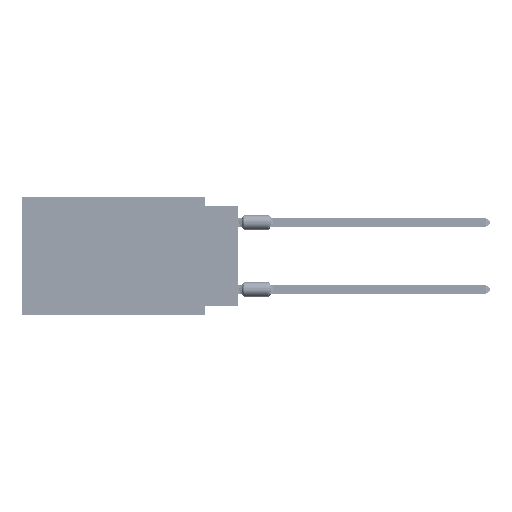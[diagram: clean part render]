
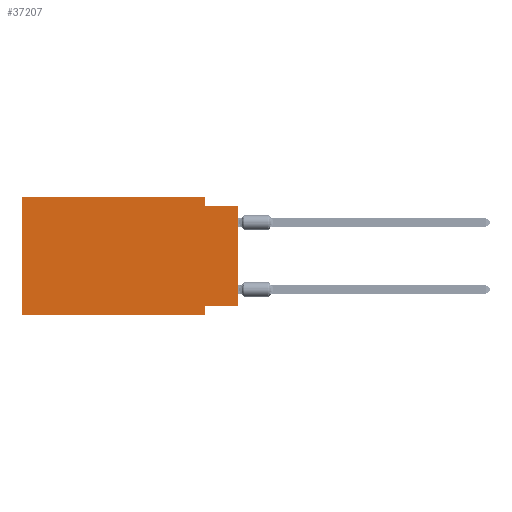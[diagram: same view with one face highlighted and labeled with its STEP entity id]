
A CAD part, left-side view. The second image highlights one B-rep face of the part: STEP entity #37207.
In plain terms, the highlighted planar face has unit normal (-1, 0, 0).
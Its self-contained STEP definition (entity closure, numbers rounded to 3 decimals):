
#640 = CARTESIAN_POINT ( 'NONE',  ( 0., 16.383, -8.89 ) ) ;
#1856 = VECTOR ( 'NONE', #93456, 1000. ) ;
#2628 = EDGE_CURVE ( 'NONE', #39612, #108847, #84671, .T. ) ;
#5478 = EDGE_CURVE ( 'NONE', #14094, #18456, #57519, .T. ) ;
#6122 = ORIENTED_EDGE ( 'NONE', *, *, #53269, .F. ) ;
#11257 = VERTEX_POINT ( 'NONE', #21645 ) ;
#11419 = CARTESIAN_POINT ( 'NONE',  ( 0., 16.383, 0. ) ) ;
#11695 = DIRECTION ( 'NONE',  ( 0., -1., 0. ) ) ;
#11996 = CARTESIAN_POINT ( 'NONE',  ( 0., 0., -8.255 ) ) ;
#14094 = VERTEX_POINT ( 'NONE', #640 ) ;
#14191 = VERTEX_POINT ( 'NONE', #103456 ) ;
#14547 = VECTOR ( 'NONE', #74507, 1000. ) ;
#17309 = VECTOR ( 'NONE', #94167, 1000. ) ;
#17633 = ORIENTED_EDGE ( 'NONE', *, *, #5478, .F. ) ;
#18456 = VERTEX_POINT ( 'NONE', #22431 ) ;
#19859 = CARTESIAN_POINT ( 'NONE',  ( 0., 16.383, 0. ) ) ;
#20325 = CARTESIAN_POINT ( 'NONE',  ( 0., 0., -0.635 ) ) ;
#20361 = CARTESIAN_POINT ( 'NONE',  ( 0., 0., -0.635 ) ) ;
#21645 = CARTESIAN_POINT ( 'NONE',  ( 0., 2.54, -8.89 ) ) ;
#22431 = CARTESIAN_POINT ( 'NONE',  ( 0., 16.383, 0. ) ) ;
#22819 = LINE ( 'NONE', #58480, #17309 ) ;
#27269 = ORIENTED_EDGE ( 'NONE', *, *, #110297, .F. ) ;
#28760 = DIRECTION ( 'NONE',  ( 0., 0., -1. ) ) ;
#29488 = DIRECTION ( 'NONE',  ( 0., 0., 1. ) ) ;
#30864 = VECTOR ( 'NONE', #11695, 1000. ) ;
#31250 = CARTESIAN_POINT ( 'NONE',  ( 0., 0., -8.255 ) ) ;
#31377 = EDGE_LOOP ( 'NONE', ( #47404, #89382, #27269, #6122, #17633, #90014, #52940, #100597 ) ) ;
#37207 = ADVANCED_FACE ( 'NONE', ( #91918 ), #108881, .F. ) ;
#39612 = VERTEX_POINT ( 'NONE', #31250 ) ;
#45721 = CARTESIAN_POINT ( 'NONE',  ( 0., 16.383, 0. ) ) ;
#46378 = DIRECTION ( 'NONE',  ( 0., 0., -1. ) ) ;
#47404 = ORIENTED_EDGE ( 'NONE', *, *, #2628, .T. ) ;
#47950 = EDGE_CURVE ( 'NONE', #14191, #108847, #65370, .T. ) ;
#52940 = ORIENTED_EDGE ( 'NONE', *, *, #88423, .F. ) ;
#53269 = EDGE_CURVE ( 'NONE', #18456, #90037, #64867, .T. ) ;
#54043 = CARTESIAN_POINT ( 'NONE',  ( 0., 2.54, -8.255 ) ) ;
#54049 = LINE ( 'NONE', #89746, #81994 ) ;
#57519 = LINE ( 'NONE', #11419, #72434 ) ;
#58480 = CARTESIAN_POINT ( 'NONE',  ( 0., 2.54, 0. ) ) ;
#64867 = LINE ( 'NONE', #19859, #30864 ) ;
#65370 = LINE ( 'NONE', #20361, #105008 ) ;
#67161 = VERTEX_POINT ( 'NONE', #54043 ) ;
#72434 = VECTOR ( 'NONE', #29488, 1000. ) ;
#72639 = AXIS2_PLACEMENT_3D ( 'NONE', #45721, #91340, #28760 ) ;
#74507 = DIRECTION ( 'NONE',  ( 0., 1., 0. ) ) ;
#81173 = DIRECTION ( 'NONE',  ( 0., -1., 0. ) ) ;
#81994 = VECTOR ( 'NONE', #108440, 1000. ) ;
#82687 = EDGE_CURVE ( 'NONE', #39612, #67161, #92082, .T. ) ;
#84671 = LINE ( 'NONE', #85247, #1856 ) ;
#85069 = CARTESIAN_POINT ( 'NONE',  ( 0., 2.54, 0. ) ) ;
#85247 = CARTESIAN_POINT ( 'NONE',  ( 0., 0., 0. ) ) ;
#88423 = EDGE_CURVE ( 'NONE', #67161, #11257, #101358, .T. ) ;
#89382 = ORIENTED_EDGE ( 'NONE', *, *, #47950, .F. ) ;
#89746 = CARTESIAN_POINT ( 'NONE',  ( 0., 16.383, -8.89 ) ) ;
#90014 = ORIENTED_EDGE ( 'NONE', *, *, #106314, .T. ) ;
#90037 = VERTEX_POINT ( 'NONE', #85069 ) ;
#91340 = DIRECTION ( 'NONE',  ( 1., 0., 0. ) ) ;
#91918 = FACE_OUTER_BOUND ( 'NONE', #31377, .T. ) ;
#92082 = LINE ( 'NONE', #11996, #14547 ) ;
#93456 = DIRECTION ( 'NONE',  ( 0., 0., 1. ) ) ;
#94167 = DIRECTION ( 'NONE',  ( 0., 0., -1. ) ) ;
#100597 = ORIENTED_EDGE ( 'NONE', *, *, #82687, .F. ) ;
#101358 = LINE ( 'NONE', #109534, #109555 ) ;
#103456 = CARTESIAN_POINT ( 'NONE',  ( 0., 2.54, -0.635 ) ) ;
#105008 = VECTOR ( 'NONE', #81173, 1000. ) ;
#106314 = EDGE_CURVE ( 'NONE', #14094, #11257, #54049, .T. ) ;
#108440 = DIRECTION ( 'NONE',  ( 0., -1., 0. ) ) ;
#108847 = VERTEX_POINT ( 'NONE', #20325 ) ;
#108881 = PLANE ( 'NONE',  #72639 ) ;
#109534 = CARTESIAN_POINT ( 'NONE',  ( 0., 2.54, -8.89 ) ) ;
#109555 = VECTOR ( 'NONE', #46378, 1000. ) ;
#110297 = EDGE_CURVE ( 'NONE', #90037, #14191, #22819, .T. ) ;
